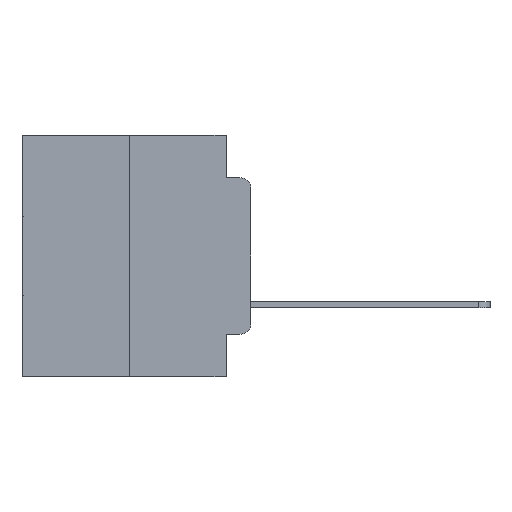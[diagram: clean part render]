
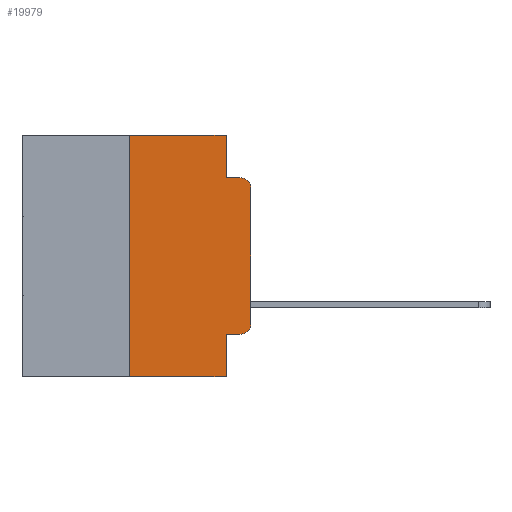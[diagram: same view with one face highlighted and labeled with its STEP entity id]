
A CAD part, left-side view. The second image highlights one B-rep face of the part: STEP entity #19979.
In plain terms, the highlighted planar face has unit normal (-1, 0, 0).
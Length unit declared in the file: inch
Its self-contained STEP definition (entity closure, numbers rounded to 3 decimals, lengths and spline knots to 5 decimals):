
#80 = EDGE_CURVE ( 'NONE', #18823, #8485, #25994, .T. ) ;
#753 = VERTEX_POINT ( 'NONE', #2882 ) ;
#783 = VERTEX_POINT ( 'NONE', #10211 ) ;
#868 = EDGE_CURVE ( 'NONE', #25437, #13932, #23831, .T. ) ;
#1055 = VECTOR ( 'NONE', #24532, 39.37008 ) ;
#1798 = CARTESIAN_POINT ( 'NONE',  ( 0., 0.02, -0.4115 ) ) ;
#2357 = EDGE_CURVE ( 'NONE', #9607, #27765, #4371, .T. ) ;
#2365 = VECTOR ( 'NONE', #12806, 39.37008 ) ;
#2538 = VECTOR ( 'NONE', #3141, 39.37008 ) ;
#2882 = CARTESIAN_POINT ( 'NONE',  ( 0., 0.25, -0.5 ) ) ;
#3106 = LINE ( 'NONE', #6719, #13373 ) ;
#3133 = ORIENTED_EDGE ( 'NONE', *, *, #11053, .F. ) ;
#3141 = DIRECTION ( 'NONE',  ( 0., 0., -1. ) ) ;
#3416 = CARTESIAN_POINT ( 'NONE',  ( 0., 0.051, 0. ) ) ;
#3488 = DIRECTION ( 'NONE',  ( 0., 0., -1. ) ) ;
#3866 = VECTOR ( 'NONE', #11913, 39.37008 ) ;
#3960 = EDGE_CURVE ( 'NONE', #20061, #8485, #20613, .T. ) ;
#4371 = CIRCLE ( 'NONE', #9926, 0.02 ) ;
#6719 = CARTESIAN_POINT ( 'NONE',  ( 0., 0.051, -0.4115 ) ) ;
#7024 = DIRECTION ( 'NONE',  ( -1., 0., 0. ) ) ;
#7465 = DIRECTION ( 'NONE',  ( -1., 0., 0. ) ) ;
#7587 = CARTESIAN_POINT ( 'NONE',  ( 0., 0.473, 0. ) ) ;
#8307 = CARTESIAN_POINT ( 'NONE',  ( 0., 0.473, 0. ) ) ;
#8485 = VERTEX_POINT ( 'NONE', #10940 ) ;
#9144 = EDGE_CURVE ( 'NONE', #27765, #18823, #22173, .T. ) ;
#9388 = CARTESIAN_POINT ( 'NONE',  ( 0., 0.02, -0.1085 ) ) ;
#9607 = VERTEX_POINT ( 'NONE', #1798 ) ;
#9775 = EDGE_CURVE ( 'NONE', #25437, #9607, #3106, .T. ) ;
#9787 = VECTOR ( 'NONE', #19040, 39.37008 ) ;
#9847 = LINE ( 'NONE', #7587, #3866 ) ;
#9926 = AXIS2_PLACEMENT_3D ( 'NONE', #16489, #7465, #12276 ) ;
#10041 = EDGE_CURVE ( 'NONE', #753, #783, #27332, .T. ) ;
#10211 = CARTESIAN_POINT ( 'NONE',  ( 0., 0.25, 0. ) ) ;
#10884 = DIRECTION ( 'NONE',  ( 0., 0., -1. ) ) ;
#10940 = CARTESIAN_POINT ( 'NONE',  ( 0., 0.02, -0.0885 ) ) ;
#11053 = EDGE_CURVE ( 'NONE', #783, #18260, #9847, .T. ) ;
#11515 = FACE_OUTER_BOUND ( 'NONE', #28345, .T. ) ;
#11913 = DIRECTION ( 'NONE',  ( 0., -1., 0. ) ) ;
#12276 = DIRECTION ( 'NONE',  ( 0., 0., -1. ) ) ;
#12499 = CARTESIAN_POINT ( 'NONE',  ( 0., 0.051, -0.0885 ) ) ;
#12527 = CARTESIAN_POINT ( 'NONE',  ( 0., 0.473, -0.5 ) ) ;
#12806 = DIRECTION ( 'NONE',  ( 0., -1., 0. ) ) ;
#12851 = EDGE_CURVE ( 'NONE', #753, #13932, #13640, .T. ) ;
#13373 = VECTOR ( 'NONE', #22425, 39.37008 ) ;
#13640 = LINE ( 'NONE', #12527, #2365 ) ;
#13932 = VERTEX_POINT ( 'NONE', #28102 ) ;
#14558 = CARTESIAN_POINT ( 'NONE',  ( 0., 0.051, 0. ) ) ;
#14934 = AXIS2_PLACEMENT_3D ( 'NONE', #8307, #24208, #10884 ) ;
#15360 = CARTESIAN_POINT ( 'NONE',  ( 0., 0.051, -0.0885 ) ) ;
#16007 = ORIENTED_EDGE ( 'NONE', *, *, #9775, .T. ) ;
#16012 = DIRECTION ( 'NONE',  ( 0., 0., 1. ) ) ;
#16489 = CARTESIAN_POINT ( 'NONE',  ( 0., 0.02, -0.3915 ) ) ;
#16690 = CARTESIAN_POINT ( 'NONE',  ( 0., 0.051, 0. ) ) ;
#16879 = ORIENTED_EDGE ( 'NONE', *, *, #9144, .T. ) ;
#18260 = VERTEX_POINT ( 'NONE', #3416 ) ;
#18561 = ORIENTED_EDGE ( 'NONE', *, *, #10041, .F. ) ;
#18823 = VERTEX_POINT ( 'NONE', #27214 ) ;
#18989 = EDGE_CURVE ( 'NONE', #18260, #20061, #28524, .T. ) ;
#19040 = DIRECTION ( 'NONE',  ( 0., 0., -1. ) ) ;
#19129 = ORIENTED_EDGE ( 'NONE', *, *, #2357, .T. ) ;
#19814 = CARTESIAN_POINT ( 'NONE',  ( 0., 0., 0. ) ) ;
#19979 = ADVANCED_FACE ( 'NONE', ( #11515 ), #21755, .F. ) ;
#20038 = CARTESIAN_POINT ( 'NONE',  ( 0., 0., -0.3915 ) ) ;
#20061 = VERTEX_POINT ( 'NONE', #15360 ) ;
#20336 = VECTOR ( 'NONE', #16012, 39.37008 ) ;
#20613 = LINE ( 'NONE', #12499, #27268 ) ;
#20662 = ORIENTED_EDGE ( 'NONE', *, *, #3960, .F. ) ;
#21755 = PLANE ( 'NONE',  #14934 ) ;
#22173 = LINE ( 'NONE', #19814, #1055 ) ;
#22314 = CARTESIAN_POINT ( 'NONE',  ( 0., 0.25, 0. ) ) ;
#22425 = DIRECTION ( 'NONE',  ( 0., -1., 0. ) ) ;
#23831 = LINE ( 'NONE', #16690, #9787 ) ;
#23838 = ORIENTED_EDGE ( 'NONE', *, *, #868, .F. ) ;
#23867 = ORIENTED_EDGE ( 'NONE', *, *, #18989, .F. ) ;
#24208 = DIRECTION ( 'NONE',  ( 1., 0., 0. ) ) ;
#24532 = DIRECTION ( 'NONE',  ( 0., 0., 1. ) ) ;
#25287 = ORIENTED_EDGE ( 'NONE', *, *, #80, .T. ) ;
#25437 = VERTEX_POINT ( 'NONE', #27189 ) ;
#25994 = CIRCLE ( 'NONE', #26598, 0.02 ) ;
#26126 = DIRECTION ( 'NONE',  ( 0., -1., 0. ) ) ;
#26598 = AXIS2_PLACEMENT_3D ( 'NONE', #9388, #7024, #3488 ) ;
#27189 = CARTESIAN_POINT ( 'NONE',  ( 0., 0.051, -0.4115 ) ) ;
#27214 = CARTESIAN_POINT ( 'NONE',  ( 0., 0., -0.1085 ) ) ;
#27268 = VECTOR ( 'NONE', #26126, 39.37008 ) ;
#27332 = LINE ( 'NONE', #22314, #20336 ) ;
#27765 = VERTEX_POINT ( 'NONE', #20038 ) ;
#28102 = CARTESIAN_POINT ( 'NONE',  ( 0., 0.051, -0.5 ) ) ;
#28345 = EDGE_LOOP ( 'NONE', ( #16879, #25287, #20662, #23867, #3133, #18561, #28996, #23838, #16007, #19129 ) ) ;
#28524 = LINE ( 'NONE', #14558, #2538 ) ;
#28996 = ORIENTED_EDGE ( 'NONE', *, *, #12851, .T. ) ;
